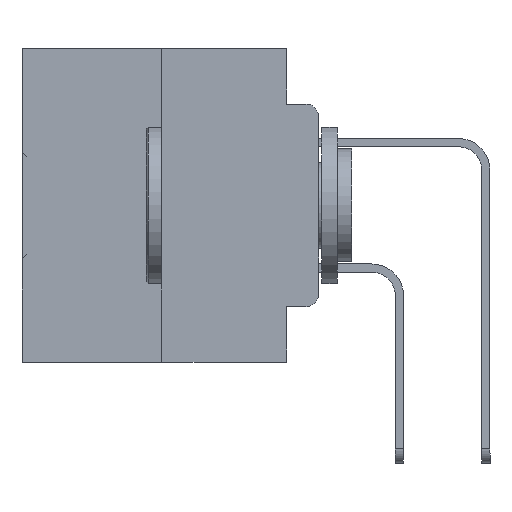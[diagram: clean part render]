
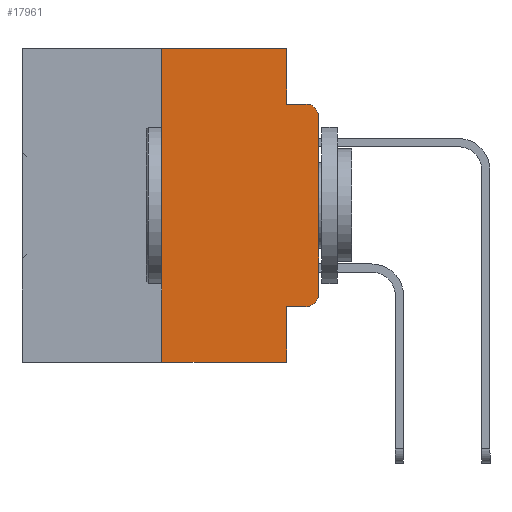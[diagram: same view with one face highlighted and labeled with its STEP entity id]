
A CAD part, left-side view. The second image highlights one B-rep face of the part: STEP entity #17961.
In plain terms, the highlighted planar face has unit normal (-1, 0, 0).
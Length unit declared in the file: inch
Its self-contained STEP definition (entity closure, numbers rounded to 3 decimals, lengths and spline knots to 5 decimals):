
#50 = CARTESIAN_POINT ( 'NONE',  ( 0., 0., -0.3915 ) ) ;
#1487 = LINE ( 'NONE', #2414, #6630 ) ;
#1541 = EDGE_CURVE ( 'NONE', #33549, #4057, #26325, .T. ) ;
#2414 = CARTESIAN_POINT ( 'NONE',  ( 0., 0.473, -0.5 ) ) ;
#3385 = VERTEX_POINT ( 'NONE', #50 ) ;
#3615 = DIRECTION ( 'NONE',  ( -1., 0., 0. ) ) ;
#3788 = VERTEX_POINT ( 'NONE', #19638 ) ;
#4057 = VERTEX_POINT ( 'NONE', #9220 ) ;
#4571 = DIRECTION ( 'NONE',  ( -1., 0., 0. ) ) ;
#4628 = CARTESIAN_POINT ( 'NONE',  ( 0., 0.25, 0. ) ) ;
#4721 = LINE ( 'NONE', #31635, #17595 ) ;
#5753 = VECTOR ( 'NONE', #7492, 39.37008 ) ;
#6017 = VECTOR ( 'NONE', #27012, 39.37008 ) ;
#6037 = CARTESIAN_POINT ( 'NONE',  ( 0., 0.051, -0.0885 ) ) ;
#6630 = VECTOR ( 'NONE', #34413, 39.37008 ) ;
#6723 = VECTOR ( 'NONE', #9322, 39.37008 ) ;
#6743 = CARTESIAN_POINT ( 'NONE',  ( 0., 0.051, 0. ) ) ;
#7492 = DIRECTION ( 'NONE',  ( 0., 0., -1. ) ) ;
#8979 = DIRECTION ( 'NONE',  ( 0., -1., 0. ) ) ;
#9220 = CARTESIAN_POINT ( 'NONE',  ( 0., 0.02, -0.0885 ) ) ;
#9322 = DIRECTION ( 'NONE',  ( 0., 0., -1. ) ) ;
#9482 = EDGE_CURVE ( 'NONE', #3385, #33549, #37570, .T. ) ;
#9577 = ORIENTED_EDGE ( 'NONE', *, *, #37231, .F. ) ;
#9583 = AXIS2_PLACEMENT_3D ( 'NONE', #21228, #3615, #24176 ) ;
#10082 = CIRCLE ( 'NONE', #9583, 0.02 ) ;
#10646 = LINE ( 'NONE', #4628, #32859 ) ;
#10801 = CARTESIAN_POINT ( 'NONE',  ( 0., 0.051, -0.5 ) ) ;
#10855 = CARTESIAN_POINT ( 'NONE',  ( 0., 0.25, -0.5 ) ) ;
#10987 = CARTESIAN_POINT ( 'NONE',  ( 0., 0.051, -0.0885 ) ) ;
#11195 = DIRECTION ( 'NONE',  ( 1., 0., 0. ) ) ;
#12603 = VERTEX_POINT ( 'NONE', #28781 ) ;
#13374 = CARTESIAN_POINT ( 'NONE',  ( 0., 0., 0. ) ) ;
#13916 = EDGE_CURVE ( 'NONE', #24832, #17373, #1487, .T. ) ;
#14612 = ORIENTED_EDGE ( 'NONE', *, *, #9482, .T. ) ;
#16020 = ORIENTED_EDGE ( 'NONE', *, *, #25947, .F. ) ;
#17373 = VERTEX_POINT ( 'NONE', #10801 ) ;
#17595 = VECTOR ( 'NONE', #34447, 39.37008 ) ;
#17870 = ORIENTED_EDGE ( 'NONE', *, *, #22029, .T. ) ;
#17961 = ADVANCED_FACE ( 'NONE', ( #23417 ), #28714, .F. ) ;
#18090 = EDGE_CURVE ( 'NONE', #33623, #3385, #10082, .T. ) ;
#19638 = CARTESIAN_POINT ( 'NONE',  ( 0., 0.051, -0.4115 ) ) ;
#20257 = AXIS2_PLACEMENT_3D ( 'NONE', #22171, #4571, #25120 ) ;
#20839 = EDGE_LOOP ( 'NONE', ( #14612, #22429, #9577, #27002, #34451, #36226, #30522, #16020, #17870, #25656 ) ) ;
#21228 = CARTESIAN_POINT ( 'NONE',  ( 0., 0.02, -0.3915 ) ) ;
#22029 = EDGE_CURVE ( 'NONE', #3788, #33623, #29322, .T. ) ;
#22171 = CARTESIAN_POINT ( 'NONE',  ( 0., 0.02, -0.1085 ) ) ;
#22291 = LINE ( 'NONE', #30628, #5753 ) ;
#22429 = ORIENTED_EDGE ( 'NONE', *, *, #1541, .T. ) ;
#22904 = CARTESIAN_POINT ( 'NONE',  ( 0., 0.473, 0. ) ) ;
#23417 = FACE_OUTER_BOUND ( 'NONE', #20839, .T. ) ;
#24176 = DIRECTION ( 'NONE',  ( 0., 0., -1. ) ) ;
#24832 = VERTEX_POINT ( 'NONE', #10855 ) ;
#24862 = VERTEX_POINT ( 'NONE', #10987 ) ;
#25120 = DIRECTION ( 'NONE',  ( 0., 0., -1. ) ) ;
#25192 = DIRECTION ( 'NONE',  ( 0., 0., 1. ) ) ;
#25656 = ORIENTED_EDGE ( 'NONE', *, *, #18090, .T. ) ;
#25947 = EDGE_CURVE ( 'NONE', #3788, #17373, #22291, .T. ) ;
#25997 = LINE ( 'NONE', #6037, #32599 ) ;
#26325 = CIRCLE ( 'NONE', #20257, 0.02 ) ;
#27002 = ORIENTED_EDGE ( 'NONE', *, *, #33484, .F. ) ;
#27012 = DIRECTION ( 'NONE',  ( 0., -1., 0. ) ) ;
#27447 = EDGE_CURVE ( 'NONE', #12603, #34166, #4721, .T. ) ;
#27885 = EDGE_CURVE ( 'NONE', #24832, #12603, #10646, .T. ) ;
#28714 = PLANE ( 'NONE',  #33582 ) ;
#28781 = CARTESIAN_POINT ( 'NONE',  ( 0., 0.25, 0. ) ) ;
#29322 = LINE ( 'NONE', #29727, #6017 ) ;
#29727 = CARTESIAN_POINT ( 'NONE',  ( 0., 0.051, -0.4115 ) ) ;
#29843 = CARTESIAN_POINT ( 'NONE',  ( 0., 0.051, 0. ) ) ;
#30161 = VECTOR ( 'NONE', #25192, 39.37008 ) ;
#30522 = ORIENTED_EDGE ( 'NONE', *, *, #13916, .T. ) ;
#30628 = CARTESIAN_POINT ( 'NONE',  ( 0., 0.051, 0. ) ) ;
#31501 = DIRECTION ( 'NONE',  ( 0., 0., -1. ) ) ;
#31635 = CARTESIAN_POINT ( 'NONE',  ( 0., 0.473, 0. ) ) ;
#32599 = VECTOR ( 'NONE', #8979, 39.37008 ) ;
#32859 = VECTOR ( 'NONE', #33564, 39.37008 ) ;
#32888 = CARTESIAN_POINT ( 'NONE',  ( 0., 0., -0.1085 ) ) ;
#33251 = CARTESIAN_POINT ( 'NONE',  ( 0., 0.02, -0.4115 ) ) ;
#33484 = EDGE_CURVE ( 'NONE', #34166, #24862, #37387, .T. ) ;
#33549 = VERTEX_POINT ( 'NONE', #32888 ) ;
#33564 = DIRECTION ( 'NONE',  ( 0., 0., 1. ) ) ;
#33582 = AXIS2_PLACEMENT_3D ( 'NONE', #22904, #11195, #31501 ) ;
#33623 = VERTEX_POINT ( 'NONE', #33251 ) ;
#34166 = VERTEX_POINT ( 'NONE', #6743 ) ;
#34413 = DIRECTION ( 'NONE',  ( 0., -1., 0. ) ) ;
#34447 = DIRECTION ( 'NONE',  ( 0., -1., 0. ) ) ;
#34451 = ORIENTED_EDGE ( 'NONE', *, *, #27447, .F. ) ;
#36226 = ORIENTED_EDGE ( 'NONE', *, *, #27885, .F. ) ;
#37231 = EDGE_CURVE ( 'NONE', #24862, #4057, #25997, .T. ) ;
#37387 = LINE ( 'NONE', #29843, #6723 ) ;
#37570 = LINE ( 'NONE', #13374, #30161 ) ;
